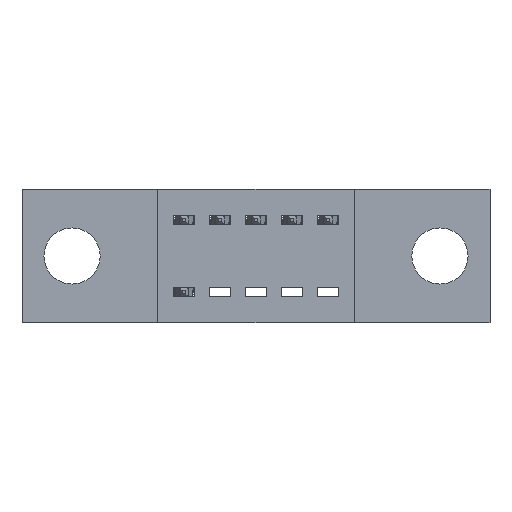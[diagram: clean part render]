
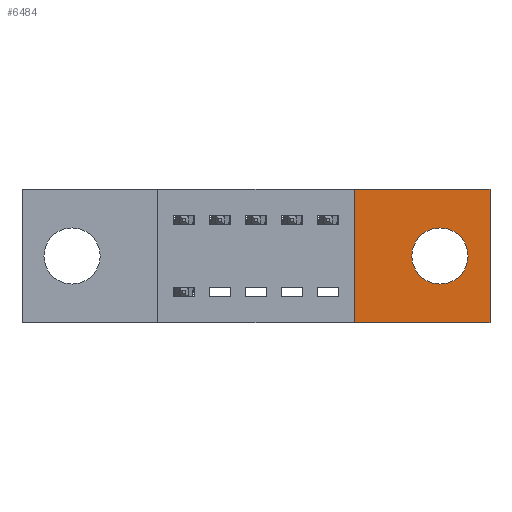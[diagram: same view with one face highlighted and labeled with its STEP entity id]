
A CAD part, front view. The second image highlights one B-rep face of the part: STEP entity #6484.
In plain terms, the highlighted planar face has unit normal (0, -1, 0).
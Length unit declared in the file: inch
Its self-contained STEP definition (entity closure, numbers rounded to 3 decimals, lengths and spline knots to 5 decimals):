
#43 = ORIENTED_EDGE ( 'NONE', *, *, #4897, .F. ) ;
#127 = CARTESIAN_POINT ( 'NONE',  ( 1.3, 0., 0. ) ) ;
#166 = ORIENTED_EDGE ( 'NONE', *, *, #3629, .F. ) ;
#651 = EDGE_CURVE ( 'NONE', #4522, #7622, #5932, .T. ) ;
#774 = VERTEX_POINT ( 'NONE', #5139 ) ;
#1322 = VECTOR ( 'NONE', #7108, 39.37008 ) ;
#1580 = VERTEX_POINT ( 'NONE', #5829 ) ;
#1640 = DIRECTION ( 'NONE',  ( -1., 0., 0. ) ) ;
#1827 = CARTESIAN_POINT ( 'NONE',  ( 0., 0., -0.37 ) ) ;
#2248 = FACE_OUTER_BOUND ( 'NONE', #7564, .T. ) ;
#2497 = CARTESIAN_POINT ( 'NONE',  ( 1.161, 0., -0.185 ) ) ;
#2603 = VECTOR ( 'NONE', #5070, 39.37008 ) ;
#2922 = CIRCLE ( 'NONE', #6703, 0.078 ) ;
#2990 = LINE ( 'NONE', #6639, #1322 ) ;
#3111 = DIRECTION ( 'NONE',  ( 0., 0., -1. ) ) ;
#3255 = EDGE_LOOP ( 'NONE', ( #5647, #5721 ) ) ;
#3629 = EDGE_CURVE ( 'NONE', #4702, #1580, #2990, .T. ) ;
#3659 = VECTOR ( 'NONE', #1640, 39.37008 ) ;
#3960 = LINE ( 'NONE', #127, #7005 ) ;
#4062 = EDGE_CURVE ( 'NONE', #774, #4702, #4375, .T. ) ;
#4086 = CARTESIAN_POINT ( 'NONE',  ( 1.161, 0., -0.185 ) ) ;
#4359 = VERTEX_POINT ( 'NONE', #4596 ) ;
#4375 = LINE ( 'NONE', #7422, #2603 ) ;
#4522 = VERTEX_POINT ( 'NONE', #7013 ) ;
#4596 = CARTESIAN_POINT ( 'NONE',  ( 1.3, 0., -0.37 ) ) ;
#4702 = VERTEX_POINT ( 'NONE', #7691 ) ;
#4897 = EDGE_CURVE ( 'NONE', #1580, #4359, #3960, .T. ) ;
#5070 = DIRECTION ( 'NONE',  ( 0., 0., 1. ) ) ;
#5103 = AXIS2_PLACEMENT_3D ( 'NONE', #4086, #6362, #6929 ) ;
#5139 = CARTESIAN_POINT ( 'NONE',  ( 0.923, 0., -0.37 ) ) ;
#5216 = DIRECTION ( 'NONE',  ( 0., 0., -1. ) ) ;
#5224 = DIRECTION ( 'NONE',  ( 0., -1., 0. ) ) ;
#5360 = PLANE ( 'NONE',  #7720 ) ;
#5390 = CARTESIAN_POINT ( 'NONE',  ( 0., 0., -0.37 ) ) ;
#5647 = ORIENTED_EDGE ( 'NONE', *, *, #7447, .T. ) ;
#5660 = FACE_BOUND ( 'NONE', #3255, .T. ) ;
#5721 = ORIENTED_EDGE ( 'NONE', *, *, #651, .T. ) ;
#5829 = CARTESIAN_POINT ( 'NONE',  ( 1.3, 0., 0. ) ) ;
#5932 = CIRCLE ( 'NONE', #5103, 0.078 ) ;
#6255 = CARTESIAN_POINT ( 'NONE',  ( 1.161, 0., -0.107 ) ) ;
#6329 = LINE ( 'NONE', #1827, #3659 ) ;
#6362 = DIRECTION ( 'NONE',  ( 0., 1., 0. ) ) ;
#6484 = ADVANCED_FACE ( 'NONE', ( #5660, #2248 ), #5360, .T. ) ;
#6639 = CARTESIAN_POINT ( 'NONE',  ( 0., 0., 0. ) ) ;
#6703 = AXIS2_PLACEMENT_3D ( 'NONE', #2497, #6722, #3111 ) ;
#6722 = DIRECTION ( 'NONE',  ( 0., 1., 0. ) ) ;
#6876 = EDGE_CURVE ( 'NONE', #4359, #774, #6329, .T. ) ;
#6929 = DIRECTION ( 'NONE',  ( 0., 0., -1. ) ) ;
#6980 = ORIENTED_EDGE ( 'NONE', *, *, #4062, .F. ) ;
#7005 = VECTOR ( 'NONE', #7051, 39.37008 ) ;
#7013 = CARTESIAN_POINT ( 'NONE',  ( 1.161, 0., -0.263 ) ) ;
#7051 = DIRECTION ( 'NONE',  ( 0., 0., -1. ) ) ;
#7108 = DIRECTION ( 'NONE',  ( 1., 0., 0. ) ) ;
#7147 = ORIENTED_EDGE ( 'NONE', *, *, #6876, .F. ) ;
#7422 = CARTESIAN_POINT ( 'NONE',  ( 0.923, 0., -0.37 ) ) ;
#7447 = EDGE_CURVE ( 'NONE', #7622, #4522, #2922, .T. ) ;
#7564 = EDGE_LOOP ( 'NONE', ( #6980, #7147, #43, #166 ) ) ;
#7622 = VERTEX_POINT ( 'NONE', #6255 ) ;
#7691 = CARTESIAN_POINT ( 'NONE',  ( 0.923, 0., 0. ) ) ;
#7720 = AXIS2_PLACEMENT_3D ( 'NONE', #5390, #5224, #5216 ) ;
